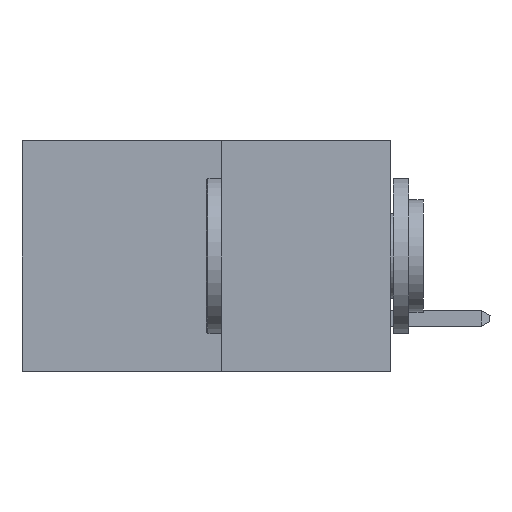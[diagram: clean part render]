
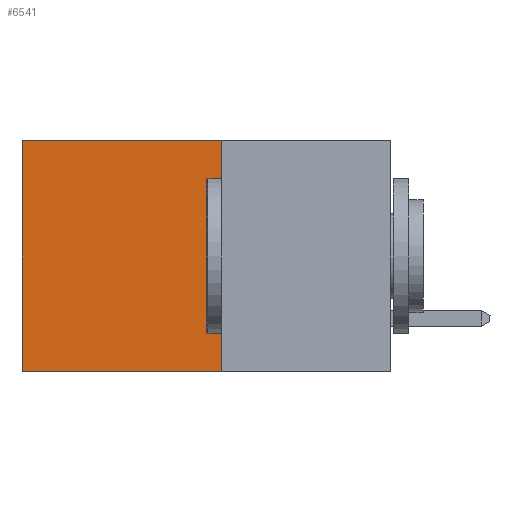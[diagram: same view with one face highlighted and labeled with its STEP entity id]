
A CAD part, left-side view. The second image highlights one B-rep face of the part: STEP entity #6541.
In plain terms, the highlighted planar face has unit normal (-1, 0, 0).
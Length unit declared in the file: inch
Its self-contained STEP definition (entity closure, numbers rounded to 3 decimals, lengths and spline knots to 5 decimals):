
#203 = LINE ( 'NONE', #10638, #16206 ) ;
#1344 = PLANE ( 'NONE',  #21361 ) ;
#2335 = CARTESIAN_POINT ( 'NONE',  ( 0.277, 0.27, 0. ) ) ;
#3156 = VERTEX_POINT ( 'NONE', #2335 ) ;
#3625 = ORIENTED_EDGE ( 'NONE', *, *, #10250, .F. ) ;
#6541 = ADVANCED_FACE ( 'NONE', ( #15328 ), #1344, .F. ) ;
#6908 = VERTEX_POINT ( 'NONE', #15649 ) ;
#6943 = CARTESIAN_POINT ( 'NONE',  ( 0.277, 0.59, -0.37 ) ) ;
#7288 = EDGE_CURVE ( 'NONE', #3156, #23623, #25473, .T. ) ;
#7948 = DIRECTION ( 'NONE',  ( 0., 0., -1. ) ) ;
#8402 = ORIENTED_EDGE ( 'NONE', *, *, #19638, .F. ) ;
#8626 = VECTOR ( 'NONE', #13072, 39.37008 ) ;
#9464 = LINE ( 'NONE', #6943, #25433 ) ;
#10245 = ORIENTED_EDGE ( 'NONE', *, *, #17313, .T. ) ;
#10250 = EDGE_CURVE ( 'NONE', #3156, #15043, #24617, .T. ) ;
#10638 = CARTESIAN_POINT ( 'NONE',  ( 0.277, 0.27, -0.37 ) ) ;
#12656 = CARTESIAN_POINT ( 'NONE',  ( 0.277, 0.27, 0. ) ) ;
#12826 = DIRECTION ( 'NONE',  ( 0., 1., 0. ) ) ;
#13072 = DIRECTION ( 'NONE',  ( 0., 0., -1. ) ) ;
#14862 = DIRECTION ( 'NONE',  ( 0., 1., 0. ) ) ;
#15043 = VERTEX_POINT ( 'NONE', #17677 ) ;
#15328 = FACE_OUTER_BOUND ( 'NONE', #23258, .T. ) ;
#15649 = CARTESIAN_POINT ( 'NONE',  ( 0.277, 0.59, -0.37 ) ) ;
#15711 = DIRECTION ( 'NONE',  ( 0., 0., -1. ) ) ;
#16206 = VECTOR ( 'NONE', #12826, 39.37008 ) ;
#17313 = EDGE_CURVE ( 'NONE', #23623, #6908, #9464, .T. ) ;
#17677 = CARTESIAN_POINT ( 'NONE',  ( 0.277, 0.27, -0.37 ) ) ;
#18317 = VECTOR ( 'NONE', #14862, 39.37008 ) ;
#18955 = ORIENTED_EDGE ( 'NONE', *, *, #7288, .T. ) ;
#19638 = EDGE_CURVE ( 'NONE', #15043, #6908, #203, .T. ) ;
#20957 = DIRECTION ( 'NONE',  ( 1., 0., 0. ) ) ;
#21361 = AXIS2_PLACEMENT_3D ( 'NONE', #27423, #20957, #7948 ) ;
#23258 = EDGE_LOOP ( 'NONE', ( #10245, #8402, #3625, #18955 ) ) ;
#23623 = VERTEX_POINT ( 'NONE', #24013 ) ;
#24013 = CARTESIAN_POINT ( 'NONE',  ( 0.277, 0.59, 0. ) ) ;
#24617 = LINE ( 'NONE', #26103, #8626 ) ;
#25433 = VECTOR ( 'NONE', #15711, 39.37008 ) ;
#25473 = LINE ( 'NONE', #12656, #18317 ) ;
#26103 = CARTESIAN_POINT ( 'NONE',  ( 0.277, 0.27, -0.37 ) ) ;
#27423 = CARTESIAN_POINT ( 'NONE',  ( 0.277, 0.27, -0.37 ) ) ;
